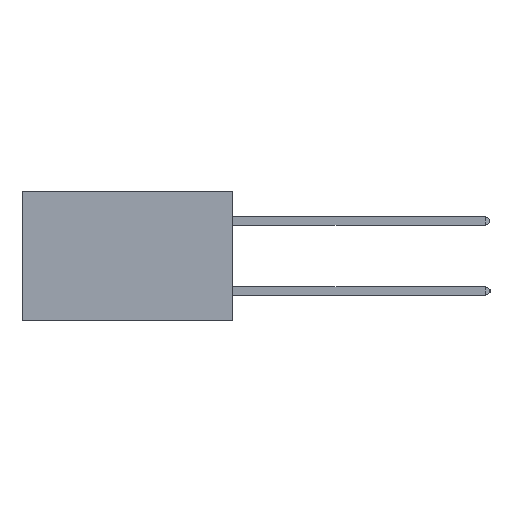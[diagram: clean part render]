
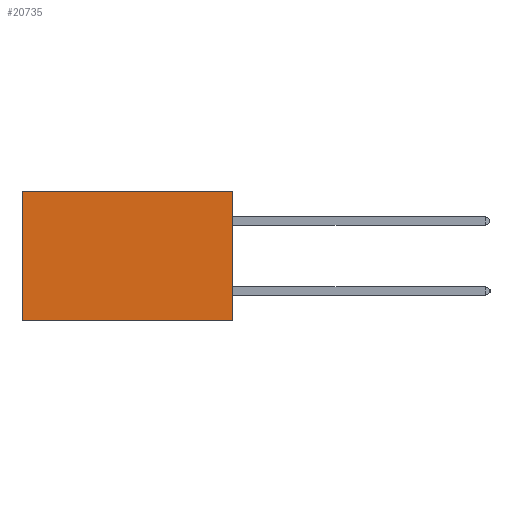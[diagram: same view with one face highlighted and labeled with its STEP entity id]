
A CAD part, left-side view. The second image highlights one B-rep face of the part: STEP entity #20735.
In plain terms, the highlighted planar face has unit normal (-1, 0, 0).
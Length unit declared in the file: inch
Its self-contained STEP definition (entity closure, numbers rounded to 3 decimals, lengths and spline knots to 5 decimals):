
#173 = DIRECTION ( 'NONE',  ( 1., 0., 0. ) ) ;
#208 = VERTEX_POINT ( 'NONE', #19910 ) ;
#1026 = CARTESIAN_POINT ( 'NONE',  ( 0.2875, 0., 0. ) ) ;
#1533 = LINE ( 'NONE', #4130, #5506 ) ;
#1793 = LINE ( 'NONE', #11449, #18323 ) ;
#1973 = ORIENTED_EDGE ( 'NONE', *, *, #9325, .F. ) ;
#2274 = VERTEX_POINT ( 'NONE', #1026 ) ;
#4130 = CARTESIAN_POINT ( 'NONE',  ( 0.2875, 0., 0. ) ) ;
#4334 = VECTOR ( 'NONE', #18559, 39.37008 ) ;
#5506 = VECTOR ( 'NONE', #10711, 39.37008 ) ;
#6892 = EDGE_CURVE ( 'NONE', #2274, #17303, #1533, .T. ) ;
#7065 = CARTESIAN_POINT ( 'NONE',  ( 0.2875, 0.6, 0. ) ) ;
#7126 = ORIENTED_EDGE ( 'NONE', *, *, #11989, .T. ) ;
#7464 = ORIENTED_EDGE ( 'NONE', *, *, #6892, .T. ) ;
#7624 = AXIS2_PLACEMENT_3D ( 'NONE', #16809, #173, #11897 ) ;
#8295 = CARTESIAN_POINT ( 'NONE',  ( 0.2875, 0.6, -0.37 ) ) ;
#9325 = EDGE_CURVE ( 'NONE', #208, #18171, #13781, .T. ) ;
#9919 = DIRECTION ( 'NONE',  ( 0., 0., -1. ) ) ;
#10711 = DIRECTION ( 'NONE',  ( 0., 1., 0. ) ) ;
#11449 = CARTESIAN_POINT ( 'NONE',  ( 0.2875, 0., 0. ) ) ;
#11897 = DIRECTION ( 'NONE',  ( 0., 0., -1. ) ) ;
#11989 = EDGE_CURVE ( 'NONE', #17303, #18171, #20182, .T. ) ;
#13247 = VECTOR ( 'NONE', #15436, 39.37008 ) ;
#13752 = CARTESIAN_POINT ( 'NONE',  ( 0.2875, 0., -0.37 ) ) ;
#13781 = LINE ( 'NONE', #13752, #13247 ) ;
#15436 = DIRECTION ( 'NONE',  ( 0., 1., 0. ) ) ;
#16809 = CARTESIAN_POINT ( 'NONE',  ( 0.2875, 0., 0. ) ) ;
#16907 = EDGE_CURVE ( 'NONE', #2274, #208, #1793, .T. ) ;
#17303 = VERTEX_POINT ( 'NONE', #19135 ) ;
#18171 = VERTEX_POINT ( 'NONE', #8295 ) ;
#18323 = VECTOR ( 'NONE', #9919, 39.37008 ) ;
#18559 = DIRECTION ( 'NONE',  ( 0., 0., -1. ) ) ;
#19135 = CARTESIAN_POINT ( 'NONE',  ( 0.2875, 0.6, 0. ) ) ;
#19160 = FACE_OUTER_BOUND ( 'NONE', #19943, .T. ) ;
#19519 = ORIENTED_EDGE ( 'NONE', *, *, #16907, .F. ) ;
#19910 = CARTESIAN_POINT ( 'NONE',  ( 0.2875, 0., -0.37 ) ) ;
#19943 = EDGE_LOOP ( 'NONE', ( #7126, #1973, #19519, #7464 ) ) ;
#19991 = PLANE ( 'NONE',  #7624 ) ;
#20182 = LINE ( 'NONE', #7065, #4334 ) ;
#20735 = ADVANCED_FACE ( 'NONE', ( #19160 ), #19991, .F. ) ;
